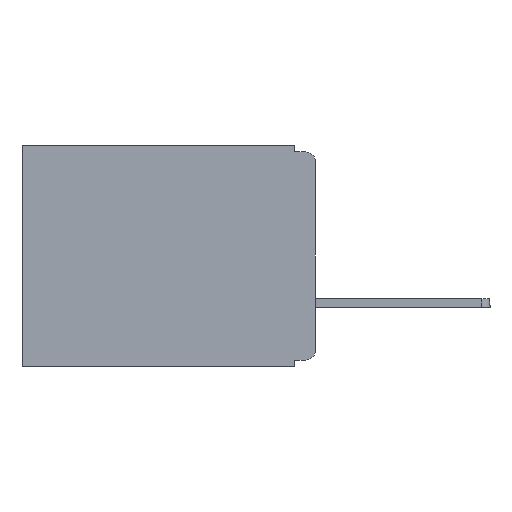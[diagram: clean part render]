
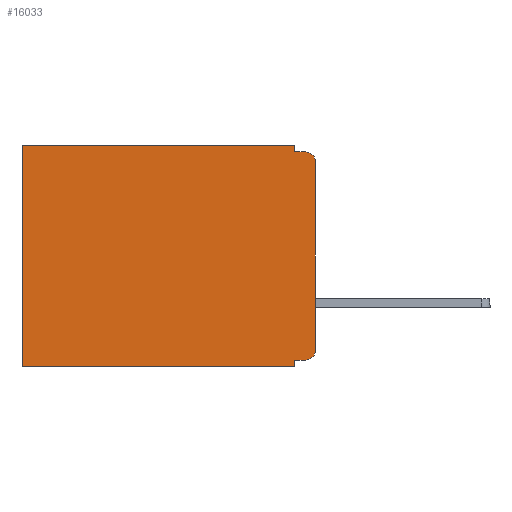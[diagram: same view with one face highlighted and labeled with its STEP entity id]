
A CAD part, left-side view. The second image highlights one B-rep face of the part: STEP entity #16033.
In plain terms, the highlighted planar face has unit normal (-1, 0, 0).
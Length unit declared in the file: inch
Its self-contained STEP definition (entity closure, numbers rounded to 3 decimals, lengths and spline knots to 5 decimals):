
#190 = DIRECTION ( 'NONE',  ( 0., 0., -1. ) ) ;
#235 = VERTEX_POINT ( 'NONE', #11286 ) ;
#440 = VECTOR ( 'NONE', #18061, 39.37008 ) ;
#697 = LINE ( 'NONE', #7907, #13290 ) ;
#1450 = EDGE_CURVE ( 'NONE', #7823, #15767, #15591, .T. ) ;
#1964 = EDGE_CURVE ( 'NONE', #5515, #17621, #7758, .T. ) ;
#2023 = CARTESIAN_POINT ( 'NONE',  ( 0.3, 0., -0.33 ) ) ;
#2246 = CARTESIAN_POINT ( 'NONE',  ( 0.3, 0., 0. ) ) ;
#2274 = ORIENTED_EDGE ( 'NONE', *, *, #1450, .F. ) ;
#2327 = CARTESIAN_POINT ( 'NONE',  ( 0.3, 0., -0.025 ) ) ;
#2460 = EDGE_CURVE ( 'NONE', #8780, #6133, #10644, .T. ) ;
#2715 = ORIENTED_EDGE ( 'NONE', *, *, #1964, .T. ) ;
#3513 = LINE ( 'NONE', #8255, #7001 ) ;
#3930 = CARTESIAN_POINT ( 'NONE',  ( 0.3, 0.437, 0. ) ) ;
#4250 = CARTESIAN_POINT ( 'NONE',  ( 0.3, 0., -0.305 ) ) ;
#4270 = DIRECTION ( 'NONE',  ( 0., 0., -1. ) ) ;
#4423 = LINE ( 'NONE', #8008, #440 ) ;
#4943 = EDGE_CURVE ( 'NONE', #12105, #235, #13692, .T. ) ;
#5008 = DIRECTION ( 'NONE',  ( 1., 0., 0. ) ) ;
#5176 = EDGE_CURVE ( 'NONE', #10987, #17479, #6222, .T. ) ;
#5347 = ORIENTED_EDGE ( 'NONE', *, *, #4943, .T. ) ;
#5515 = VERTEX_POINT ( 'NONE', #16523 ) ;
#5807 = CARTESIAN_POINT ( 'NONE',  ( 0.3, 0.031, 0. ) ) ;
#5830 = ORIENTED_EDGE ( 'NONE', *, *, #10880, .T. ) ;
#6112 = DIRECTION ( 'NONE',  ( 0., 0., -1. ) ) ;
#6133 = VERTEX_POINT ( 'NONE', #14319 ) ;
#6222 = LINE ( 'NONE', #7607, #13466 ) ;
#6231 = EDGE_LOOP ( 'NONE', ( #12596, #5347, #9271, #16919, #5830, #9725, #12803, #2274, #6541, #2715 ) ) ;
#6321 = CARTESIAN_POINT ( 'NONE',  ( 0.3, 0.031, -0.33 ) ) ;
#6541 = ORIENTED_EDGE ( 'NONE', *, *, #10808, .F. ) ;
#6761 = DIRECTION ( 'NONE',  ( 0., 1., 0. ) ) ;
#6811 = VECTOR ( 'NONE', #4270, 39.37008 ) ;
#7001 = VECTOR ( 'NONE', #6761, 39.37008 ) ;
#7417 = VECTOR ( 'NONE', #12431, 39.37008 ) ;
#7588 = DIRECTION ( 'NONE',  ( 0., 0., -1. ) ) ;
#7607 = CARTESIAN_POINT ( 'NONE',  ( 0.3, 0.437, -0.33 ) ) ;
#7758 = CIRCLE ( 'NONE', #13465, 0.015 ) ;
#7823 = VERTEX_POINT ( 'NONE', #16704 ) ;
#7907 = CARTESIAN_POINT ( 'NONE',  ( 0.3, 0., -0.33 ) ) ;
#8008 = CARTESIAN_POINT ( 'NONE',  ( 0.3, 0., -0.32 ) ) ;
#8255 = CARTESIAN_POINT ( 'NONE',  ( 0.3, 0., -0.33 ) ) ;
#8780 = VERTEX_POINT ( 'NONE', #8835 ) ;
#8835 = CARTESIAN_POINT ( 'NONE',  ( 0.3, 0.031, 0. ) ) ;
#9170 = DIRECTION ( 'NONE',  ( 0., -1., 0. ) ) ;
#9208 = AXIS2_PLACEMENT_3D ( 'NONE', #2023, #5008, #15125 ) ;
#9271 = ORIENTED_EDGE ( 'NONE', *, *, #16597, .F. ) ;
#9502 = EDGE_CURVE ( 'NONE', #12105, #17621, #697, .T. ) ;
#9725 = ORIENTED_EDGE ( 'NONE', *, *, #5176, .T. ) ;
#10052 = AXIS2_PLACEMENT_3D ( 'NONE', #16736, #13749, #13728 ) ;
#10257 = VECTOR ( 'NONE', #9170, 39.37008 ) ;
#10644 = LINE ( 'NONE', #5807, #6811 ) ;
#10734 = DIRECTION ( 'NONE',  ( 0., 0., -1. ) ) ;
#10808 = EDGE_CURVE ( 'NONE', #5515, #7823, #4423, .T. ) ;
#10880 = EDGE_CURVE ( 'NONE', #8780, #10987, #18001, .T. ) ;
#10987 = VERTEX_POINT ( 'NONE', #3930 ) ;
#11286 = CARTESIAN_POINT ( 'NONE',  ( 0.3, 0.015, -0.01 ) ) ;
#11785 = CARTESIAN_POINT ( 'NONE',  ( 0.3, 0.015, -0.305 ) ) ;
#12105 = VERTEX_POINT ( 'NONE', #2327 ) ;
#12431 = DIRECTION ( 'NONE',  ( 0., 1., 0. ) ) ;
#12596 = ORIENTED_EDGE ( 'NONE', *, *, #9502, .F. ) ;
#12803 = ORIENTED_EDGE ( 'NONE', *, *, #13208, .F. ) ;
#12964 = FACE_OUTER_BOUND ( 'NONE', #6231, .T. ) ;
#13208 = EDGE_CURVE ( 'NONE', #15767, #17479, #3513, .T. ) ;
#13290 = VECTOR ( 'NONE', #10734, 39.37008 ) ;
#13422 = DIRECTION ( 'NONE',  ( -1., 0., 0. ) ) ;
#13465 = AXIS2_PLACEMENT_3D ( 'NONE', #11785, #13422, #190 ) ;
#13466 = VECTOR ( 'NONE', #7588, 39.37008 ) ;
#13692 = CIRCLE ( 'NONE', #10052, 0.015 ) ;
#13728 = DIRECTION ( 'NONE',  ( 0., 0., -1. ) ) ;
#13749 = DIRECTION ( 'NONE',  ( -1., 0., 0. ) ) ;
#14049 = LINE ( 'NONE', #16306, #10257 ) ;
#14254 = CARTESIAN_POINT ( 'NONE',  ( 0.3, 0.031, -0.33 ) ) ;
#14319 = CARTESIAN_POINT ( 'NONE',  ( 0.3, 0.031, -0.01 ) ) ;
#15125 = DIRECTION ( 'NONE',  ( 0., 0., -1. ) ) ;
#15135 = VECTOR ( 'NONE', #6112, 39.37008 ) ;
#15452 = CARTESIAN_POINT ( 'NONE',  ( 0.3, 0.437, -0.33 ) ) ;
#15591 = LINE ( 'NONE', #6321, #15135 ) ;
#15767 = VERTEX_POINT ( 'NONE', #14254 ) ;
#16033 = ADVANCED_FACE ( 'NONE', ( #12964 ), #17987, .F. ) ;
#16306 = CARTESIAN_POINT ( 'NONE',  ( 0.3, 0., -0.01 ) ) ;
#16523 = CARTESIAN_POINT ( 'NONE',  ( 0.3, 0.015, -0.32 ) ) ;
#16597 = EDGE_CURVE ( 'NONE', #6133, #235, #14049, .T. ) ;
#16704 = CARTESIAN_POINT ( 'NONE',  ( 0.3, 0.031, -0.32 ) ) ;
#16736 = CARTESIAN_POINT ( 'NONE',  ( 0.3, 0.015, -0.025 ) ) ;
#16919 = ORIENTED_EDGE ( 'NONE', *, *, #2460, .F. ) ;
#17479 = VERTEX_POINT ( 'NONE', #15452 ) ;
#17621 = VERTEX_POINT ( 'NONE', #4250 ) ;
#17987 = PLANE ( 'NONE',  #9208 ) ;
#18001 = LINE ( 'NONE', #2246, #7417 ) ;
#18061 = DIRECTION ( 'NONE',  ( 0., 1., 0. ) ) ;
